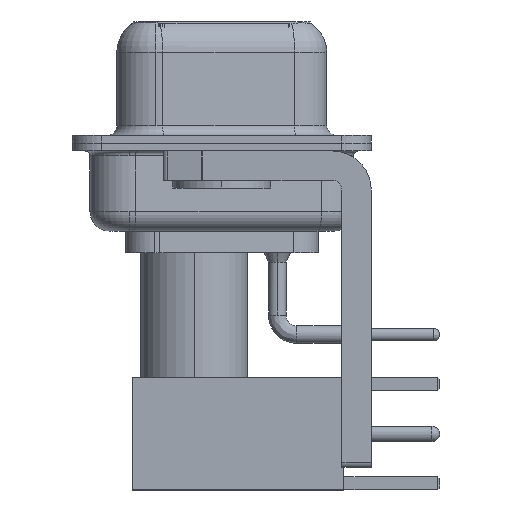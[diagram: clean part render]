
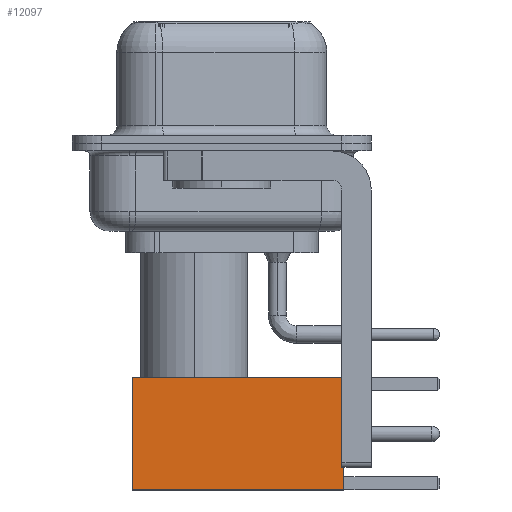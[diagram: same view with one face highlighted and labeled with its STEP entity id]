
A CAD part, left-side view. The second image highlights one B-rep face of the part: STEP entity #12097.
In plain terms, the highlighted face is planar.
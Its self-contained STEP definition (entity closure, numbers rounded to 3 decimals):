
#484 = VERTEX_POINT ( 'NONE', #12752 ) ;
#529 = CARTESIAN_POINT ( 'NONE',  ( 2.875, 2.875, 0. ) ) ;
#1101 = VECTOR ( 'NONE', #12705, 1000. ) ;
#1184 = CARTESIAN_POINT ( 'NONE',  ( 0., 2.875, 0. ) ) ;
#1588 = CARTESIAN_POINT ( 'NONE',  ( -2.875, 2.875, 0. ) ) ;
#2565 = CARTESIAN_POINT ( 'NONE',  ( -2.875, 2.875, 0. ) ) ;
#4613 = CARTESIAN_POINT ( 'NONE',  ( 0., 2.875, 10.82 ) ) ;
#6416 = VERTEX_POINT ( 'NONE', #1588 ) ;
#7633 = EDGE_CURVE ( 'NONE', #484, #18139, #17334, .T. ) ;
#7744 = VECTOR ( 'NONE', #10780, 1000. ) ;
#7950 = VECTOR ( 'NONE', #17067, 1000. ) ;
#9161 = LINE ( 'NONE', #1184, #20317 ) ;
#9862 = AXIS2_PLACEMENT_3D ( 'NONE', #16450, #24714, #26343 ) ;
#10780 = DIRECTION ( 'NONE',  ( 0., 0., -1. ) ) ;
#11521 = ORIENTED_EDGE ( 'NONE', *, *, #7633, .F. ) ;
#12097 = ADVANCED_FACE ( 'NONE', ( #13999 ), #22281, .T. ) ;
#12187 = CARTESIAN_POINT ( 'NONE',  ( -2.875, 2.875, 10.82 ) ) ;
#12705 = DIRECTION ( 'NONE',  ( -1., 0., 0. ) ) ;
#12752 = CARTESIAN_POINT ( 'NONE',  ( 2.875, 2.875, 10.82 ) ) ;
#13203 = EDGE_CURVE ( 'NONE', #18139, #6416, #20841, .T. ) ;
#13331 = EDGE_CURVE ( 'NONE', #23083, #6416, #9161, .T. ) ;
#13375 = CARTESIAN_POINT ( 'NONE',  ( 2.875, 2.875, 0. ) ) ;
#13999 = FACE_OUTER_BOUND ( 'NONE', #23963, .T. ) ;
#16450 = CARTESIAN_POINT ( 'NONE',  ( 2.875, 2.875, 0. ) ) ;
#17067 = DIRECTION ( 'NONE',  ( 0., 0., -1. ) ) ;
#17334 = LINE ( 'NONE', #4613, #1101 ) ;
#18139 = VERTEX_POINT ( 'NONE', #12187 ) ;
#20317 = VECTOR ( 'NONE', #25972, 1000. ) ;
#20841 = LINE ( 'NONE', #2565, #7744 ) ;
#21389 = LINE ( 'NONE', #529, #7950 ) ;
#21671 = ORIENTED_EDGE ( 'NONE', *, *, #13203, .F. ) ;
#22281 = PLANE ( 'NONE',  #9862 ) ;
#22958 = EDGE_CURVE ( 'NONE', #484, #23083, #21389, .T. ) ;
#23083 = VERTEX_POINT ( 'NONE', #13375 ) ;
#23963 = EDGE_LOOP ( 'NONE', ( #26495, #24475, #21671, #11521 ) ) ;
#24475 = ORIENTED_EDGE ( 'NONE', *, *, #13331, .T. ) ;
#24714 = DIRECTION ( 'NONE',  ( 0., 1., 0. ) ) ;
#25972 = DIRECTION ( 'NONE',  ( -1., 0., 0. ) ) ;
#26343 = DIRECTION ( 'NONE',  ( 0., 0., 1. ) ) ;
#26495 = ORIENTED_EDGE ( 'NONE', *, *, #22958, .T. ) ;
